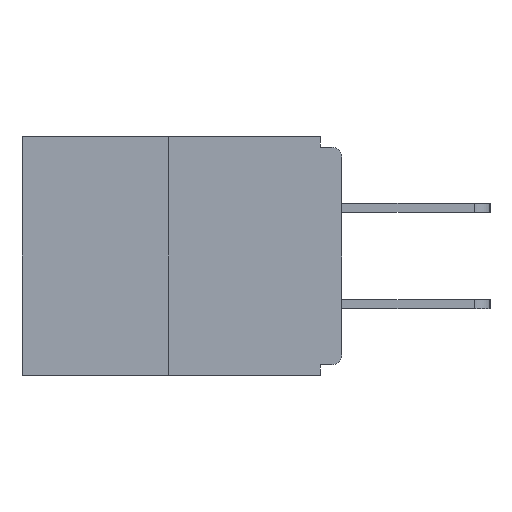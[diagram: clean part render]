
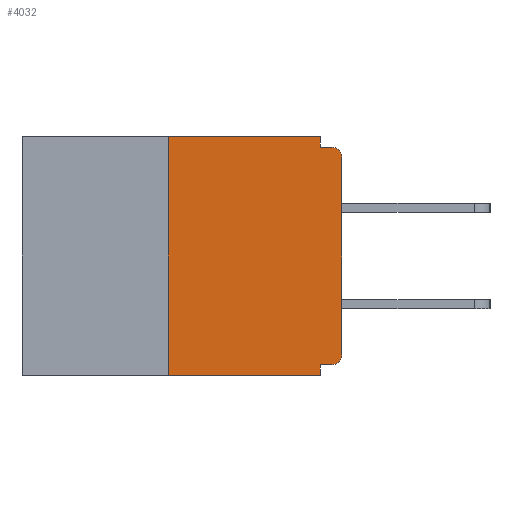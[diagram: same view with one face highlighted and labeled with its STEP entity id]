
A CAD part, left-side view. The second image highlights one B-rep face of the part: STEP entity #4032.
In plain terms, the highlighted planar face has unit normal (-1, 0, 0).
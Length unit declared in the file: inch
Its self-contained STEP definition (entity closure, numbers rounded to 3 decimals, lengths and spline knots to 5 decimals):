
#1028 = VECTOR ( 'NONE', #2977, 39.37008 ) ;
#1107 = LINE ( 'NONE', #6277, #26516 ) ;
#1288 = DIRECTION ( 'NONE',  ( 1., 0., 0. ) ) ;
#1330 = CARTESIAN_POINT ( 'NONE',  ( 0., 0.015, -0.03 ) ) ;
#1426 = CARTESIAN_POINT ( 'NONE',  ( 0., 0.25, -0.343 ) ) ;
#2063 = FACE_OUTER_BOUND ( 'NONE', #24196, .T. ) ;
#2172 = EDGE_CURVE ( 'NONE', #13174, #6363, #12065, .T. ) ;
#2422 = LINE ( 'NONE', #9577, #1028 ) ;
#2911 = AXIS2_PLACEMENT_3D ( 'NONE', #1330, #26185, #19657 ) ;
#2977 = DIRECTION ( 'NONE',  ( 0., -1., 0. ) ) ;
#3074 = VERTEX_POINT ( 'NONE', #15172 ) ;
#3970 = CARTESIAN_POINT ( 'NONE',  ( 0., 0., -0.328 ) ) ;
#4032 = ADVANCED_FACE ( 'NONE', ( #2063 ), #14994, .F. ) ;
#4316 = VERTEX_POINT ( 'NONE', #14505 ) ;
#4590 = CARTESIAN_POINT ( 'NONE',  ( 0., 0.031, -0.343 ) ) ;
#5231 = VERTEX_POINT ( 'NONE', #23952 ) ;
#5548 = AXIS2_PLACEMENT_3D ( 'NONE', #20179, #22370, #8946 ) ;
#5999 = CARTESIAN_POINT ( 'NONE',  ( 0., 0.031, -0.328 ) ) ;
#6219 = LINE ( 'NONE', #10218, #20710 ) ;
#6277 = CARTESIAN_POINT ( 'NONE',  ( 0., 0.031, 0. ) ) ;
#6363 = VERTEX_POINT ( 'NONE', #5999 ) ;
#6416 = EDGE_CURVE ( 'NONE', #4316, #8701, #1107, .T. ) ;
#6585 = CARTESIAN_POINT ( 'NONE',  ( 0., 0., 0. ) ) ;
#7023 = LINE ( 'NONE', #6585, #26482 ) ;
#7180 = ORIENTED_EDGE ( 'NONE', *, *, #22031, .F. ) ;
#7326 = LINE ( 'NONE', #17381, #7679 ) ;
#7572 = VERTEX_POINT ( 'NONE', #14310 ) ;
#7679 = VECTOR ( 'NONE', #26564, 39.37008 ) ;
#7888 = EDGE_CURVE ( 'NONE', #19596, #7572, #2422, .T. ) ;
#8237 = EDGE_CURVE ( 'NONE', #19596, #14750, #7326, .T. ) ;
#8701 = VERTEX_POINT ( 'NONE', #16370 ) ;
#8802 = EDGE_CURVE ( 'NONE', #14750, #4316, #23187, .T. ) ;
#8946 = DIRECTION ( 'NONE',  ( 0., 0., -1. ) ) ;
#9577 = CARTESIAN_POINT ( 'NONE',  ( 0., 0.46, -0.343 ) ) ;
#10157 = DIRECTION ( 'NONE',  ( 0., 1., 0. ) ) ;
#10218 = CARTESIAN_POINT ( 'NONE',  ( 0., 0., -0.015 ) ) ;
#10455 = AXIS2_PLACEMENT_3D ( 'NONE', #19222, #1288, #25868 ) ;
#11859 = ORIENTED_EDGE ( 'NONE', *, *, #2172, .F. ) ;
#12065 = LINE ( 'NONE', #3970, #13812 ) ;
#12244 = ORIENTED_EDGE ( 'NONE', *, *, #7888, .T. ) ;
#12329 = VECTOR ( 'NONE', #24628, 39.37008 ) ;
#12352 = ORIENTED_EDGE ( 'NONE', *, *, #20256, .T. ) ;
#12392 = DIRECTION ( 'NONE',  ( 0., -1., 0. ) ) ;
#12412 = DIRECTION ( 'NONE',  ( 0., -1., 0. ) ) ;
#12728 = CARTESIAN_POINT ( 'NONE',  ( 0., 0.015, -0.328 ) ) ;
#13174 = VERTEX_POINT ( 'NONE', #12728 ) ;
#13444 = CARTESIAN_POINT ( 'NONE',  ( 0., 0., -0.03 ) ) ;
#13812 = VECTOR ( 'NONE', #10157, 39.37008 ) ;
#13889 = CARTESIAN_POINT ( 'NONE',  ( 0., 0.25, 0. ) ) ;
#14310 = CARTESIAN_POINT ( 'NONE',  ( 0., 0.031, -0.343 ) ) ;
#14505 = CARTESIAN_POINT ( 'NONE',  ( 0., 0.031, 0. ) ) ;
#14750 = VERTEX_POINT ( 'NONE', #13889 ) ;
#14994 = PLANE ( 'NONE',  #10455 ) ;
#15172 = CARTESIAN_POINT ( 'NONE',  ( 0., 0.015, -0.015 ) ) ;
#15481 = CIRCLE ( 'NONE', #2911, 0.015 ) ;
#15722 = DIRECTION ( 'NONE',  ( 0., 0., 1. ) ) ;
#16151 = EDGE_CURVE ( 'NONE', #13174, #5231, #25243, .T. ) ;
#16370 = CARTESIAN_POINT ( 'NONE',  ( 0., 0.031, -0.015 ) ) ;
#16749 = ORIENTED_EDGE ( 'NONE', *, *, #6416, .F. ) ;
#17181 = VECTOR ( 'NONE', #12392, 39.37008 ) ;
#17381 = CARTESIAN_POINT ( 'NONE',  ( 0., 0.25, 0. ) ) ;
#18496 = CARTESIAN_POINT ( 'NONE',  ( 0., 0.46, 0. ) ) ;
#19222 = CARTESIAN_POINT ( 'NONE',  ( 0., 0.46, 0. ) ) ;
#19596 = VERTEX_POINT ( 'NONE', #1426 ) ;
#19657 = DIRECTION ( 'NONE',  ( 0., 0., -1. ) ) ;
#20179 = CARTESIAN_POINT ( 'NONE',  ( 0., 0.015, -0.313 ) ) ;
#20256 = EDGE_CURVE ( 'NONE', #5231, #22773, #7023, .T. ) ;
#20413 = ORIENTED_EDGE ( 'NONE', *, *, #21688, .T. ) ;
#20710 = VECTOR ( 'NONE', #12412, 39.37008 ) ;
#21688 = EDGE_CURVE ( 'NONE', #22773, #3074, #15481, .T. ) ;
#22031 = EDGE_CURVE ( 'NONE', #8701, #3074, #6219, .T. ) ;
#22095 = ORIENTED_EDGE ( 'NONE', *, *, #16151, .T. ) ;
#22370 = DIRECTION ( 'NONE',  ( -1., 0., 0. ) ) ;
#22773 = VERTEX_POINT ( 'NONE', #13444 ) ;
#23187 = LINE ( 'NONE', #18496, #17181 ) ;
#23952 = CARTESIAN_POINT ( 'NONE',  ( 0., 0., -0.313 ) ) ;
#24196 = EDGE_LOOP ( 'NONE', ( #27302, #24429, #12244, #24622, #11859, #22095, #12352, #20413, #7180, #16749 ) ) ;
#24429 = ORIENTED_EDGE ( 'NONE', *, *, #8237, .F. ) ;
#24622 = ORIENTED_EDGE ( 'NONE', *, *, #28576, .F. ) ;
#24628 = DIRECTION ( 'NONE',  ( 0., 0., -1. ) ) ;
#25243 = CIRCLE ( 'NONE', #5548, 0.015 ) ;
#25868 = DIRECTION ( 'NONE',  ( 0., 0., -1. ) ) ;
#26185 = DIRECTION ( 'NONE',  ( -1., 0., 0. ) ) ;
#26482 = VECTOR ( 'NONE', #15722, 39.37008 ) ;
#26516 = VECTOR ( 'NONE', #29107, 39.37008 ) ;
#26564 = DIRECTION ( 'NONE',  ( 0., 0., 1. ) ) ;
#27302 = ORIENTED_EDGE ( 'NONE', *, *, #8802, .F. ) ;
#27551 = LINE ( 'NONE', #4590, #12329 ) ;
#28576 = EDGE_CURVE ( 'NONE', #6363, #7572, #27551, .T. ) ;
#29107 = DIRECTION ( 'NONE',  ( 0., 0., -1. ) ) ;
